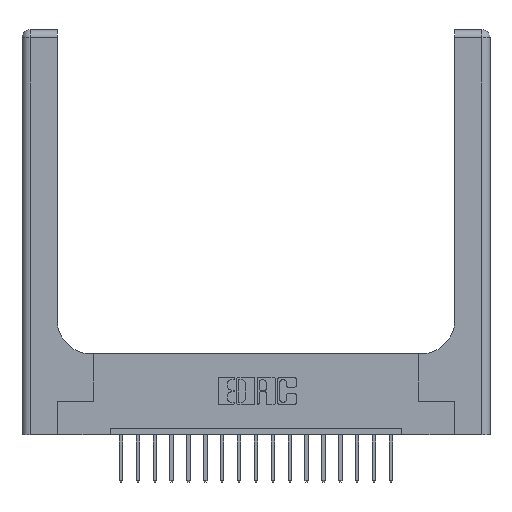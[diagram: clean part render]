
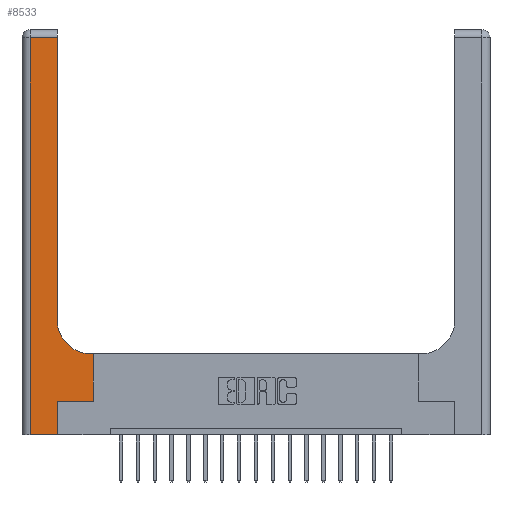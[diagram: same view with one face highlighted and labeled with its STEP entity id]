
A CAD part, top view. The second image highlights one B-rep face of the part: STEP entity #8533.
In plain terms, the highlighted planar face has unit normal (0, 0, 1).
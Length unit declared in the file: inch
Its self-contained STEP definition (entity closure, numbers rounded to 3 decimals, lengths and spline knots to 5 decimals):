
#115 = CARTESIAN_POINT ( 'NONE',  ( 0.528, 0.6, 0.37 ) ) ;
#342 = EDGE_CURVE ( 'NONE', #15315, #6598, #5647, .T. ) ;
#369 = EDGE_CURVE ( 'NONE', #1947, #13411, #7220, .T. ) ;
#395 = LINE ( 'NONE', #13648, #17017 ) ;
#676 = LINE ( 'NONE', #7756, #7138 ) ;
#874 = ORIENTED_EDGE ( 'NONE', *, *, #342, .T. ) ;
#1343 = LINE ( 'NONE', #17232, #9885 ) ;
#1495 = CARTESIAN_POINT ( 'NONE',  ( 0.51, 0.85, 0.37 ) ) ;
#1947 = VERTEX_POINT ( 'NONE', #8592 ) ;
#2098 = EDGE_CURVE ( 'NONE', #6598, #12839, #1343, .T. ) ;
#2391 = FACE_OUTER_BOUND ( 'NONE', #12151, .T. ) ;
#2653 = VERTEX_POINT ( 'NONE', #8149 ) ;
#2826 = ORIENTED_EDGE ( 'NONE', *, *, #15422, .T. ) ;
#3101 = LINE ( 'NONE', #11870, #8891 ) ;
#3594 = CARTESIAN_POINT ( 'NONE',  ( 0.06, 0., 0.37 ) ) ;
#3748 = CARTESIAN_POINT ( 'NONE',  ( 0.06, 2.94, 0.37 ) ) ;
#3919 = EDGE_CURVE ( 'NONE', #2653, #7316, #676, .T. ) ;
#4327 = DIRECTION ( 'NONE',  ( 0., 1., 0. ) ) ;
#4618 = CARTESIAN_POINT ( 'NONE',  ( 0.265, 0., 0.37 ) ) ;
#5358 = DIRECTION ( 'NONE',  ( 1., 0., 0. ) ) ;
#5647 = LINE ( 'NONE', #7370, #11607 ) ;
#6156 = CARTESIAN_POINT ( 'NONE',  ( 0.26, 0.85, 0.37 ) ) ;
#6598 = VERTEX_POINT ( 'NONE', #3748 ) ;
#7138 = VECTOR ( 'NONE', #14890, 39.37008 ) ;
#7187 = DIRECTION ( 'NONE',  ( 0., 0., -1. ) ) ;
#7220 = CIRCLE ( 'NONE', #12725, 0.25 ) ;
#7246 = DIRECTION ( 'NONE',  ( -1., 0., 0. ) ) ;
#7316 = VERTEX_POINT ( 'NONE', #115 ) ;
#7364 = DIRECTION ( 'NONE',  ( -1., 0., 0. ) ) ;
#7370 = CARTESIAN_POINT ( 'NONE',  ( 0., 2.94, 0.37 ) ) ;
#7622 = VECTOR ( 'NONE', #9147, 39.37008 ) ;
#7624 = EDGE_CURVE ( 'NONE', #13411, #15315, #13510, .T. ) ;
#7756 = CARTESIAN_POINT ( 'NONE',  ( 0.528, 0.25, 0.37 ) ) ;
#7771 = PLANE ( 'NONE',  #13806 ) ;
#8149 = CARTESIAN_POINT ( 'NONE',  ( 0.528, 0.25, 0.37 ) ) ;
#8208 = DIRECTION ( 'NONE',  ( 1., 0., 0. ) ) ;
#8533 = ADVANCED_FACE ( 'NONE', ( #2391 ), #7771, .F. ) ;
#8592 = CARTESIAN_POINT ( 'NONE',  ( 0.51, 0.6, 0.37 ) ) ;
#8699 = CARTESIAN_POINT ( 'NONE',  ( 0.26, 3., 0.37 ) ) ;
#8891 = VECTOR ( 'NONE', #7364, 39.37008 ) ;
#9043 = CARTESIAN_POINT ( 'NONE',  ( 0.265, 0.25, 0.37 ) ) ;
#9076 = ORIENTED_EDGE ( 'NONE', *, *, #369, .T. ) ;
#9147 = DIRECTION ( 'NONE',  ( 0., 1., 0. ) ) ;
#9151 = ORIENTED_EDGE ( 'NONE', *, *, #10660, .T. ) ;
#9788 = DIRECTION ( 'NONE',  ( 0., 0., -1. ) ) ;
#9885 = VECTOR ( 'NONE', #9985, 39.37008 ) ;
#9985 = DIRECTION ( 'NONE',  ( 0., -1., 0. ) ) ;
#10301 = VERTEX_POINT ( 'NONE', #9043 ) ;
#10302 = ORIENTED_EDGE ( 'NONE', *, *, #7624, .T. ) ;
#10468 = CARTESIAN_POINT ( 'NONE',  ( 0., 3., 0.37 ) ) ;
#10660 = EDGE_CURVE ( 'NONE', #18764, #10301, #14706, .T. ) ;
#10907 = CARTESIAN_POINT ( 'NONE',  ( 0.265, 0.25, 0.37 ) ) ;
#11358 = ORIENTED_EDGE ( 'NONE', *, *, #2098, .T. ) ;
#11607 = VECTOR ( 'NONE', #7246, 39.37008 ) ;
#11870 = CARTESIAN_POINT ( 'NONE',  ( 0.26, 0.6, 0.37 ) ) ;
#12151 = EDGE_LOOP ( 'NONE', ( #10302, #874, #11358, #12437, #9151, #2826, #14657, #14997, #9076 ) ) ;
#12437 = ORIENTED_EDGE ( 'NONE', *, *, #13581, .T. ) ;
#12725 = AXIS2_PLACEMENT_3D ( 'NONE', #1495, #7187, #13228 ) ;
#12839 = VERTEX_POINT ( 'NONE', #3594 ) ;
#13228 = DIRECTION ( 'NONE',  ( 1., 0., 0. ) ) ;
#13411 = VERTEX_POINT ( 'NONE', #6156 ) ;
#13510 = LINE ( 'NONE', #8699, #17227 ) ;
#13581 = EDGE_CURVE ( 'NONE', #12839, #18764, #395, .T. ) ;
#13648 = CARTESIAN_POINT ( 'NONE',  ( 0., 0., 0.37 ) ) ;
#13806 = AXIS2_PLACEMENT_3D ( 'NONE', #10468, #9788, #15786 ) ;
#13929 = LINE ( 'NONE', #10907, #17387 ) ;
#14056 = EDGE_CURVE ( 'NONE', #7316, #1947, #3101, .T. ) ;
#14657 = ORIENTED_EDGE ( 'NONE', *, *, #3919, .T. ) ;
#14706 = LINE ( 'NONE', #4618, #7622 ) ;
#14890 = DIRECTION ( 'NONE',  ( 0., 1., 0. ) ) ;
#14997 = ORIENTED_EDGE ( 'NONE', *, *, #14056, .T. ) ;
#15315 = VERTEX_POINT ( 'NONE', #18296 ) ;
#15422 = EDGE_CURVE ( 'NONE', #10301, #2653, #13929, .T. ) ;
#15786 = DIRECTION ( 'NONE',  ( -1., 0., 0. ) ) ;
#17017 = VECTOR ( 'NONE', #8208, 39.37008 ) ;
#17227 = VECTOR ( 'NONE', #4327, 39.37008 ) ;
#17232 = CARTESIAN_POINT ( 'NONE',  ( 0.06, 3., 0.37 ) ) ;
#17387 = VECTOR ( 'NONE', #5358, 39.37008 ) ;
#18296 = CARTESIAN_POINT ( 'NONE',  ( 0.26, 2.94, 0.37 ) ) ;
#18764 = VERTEX_POINT ( 'NONE', #18939 ) ;
#18939 = CARTESIAN_POINT ( 'NONE',  ( 0.265, 0., 0.37 ) ) ;
